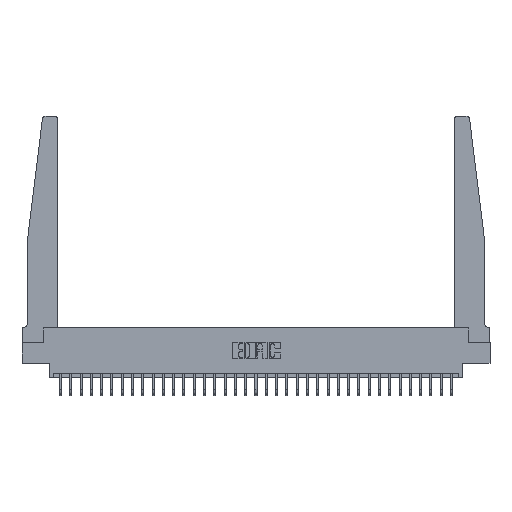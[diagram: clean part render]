
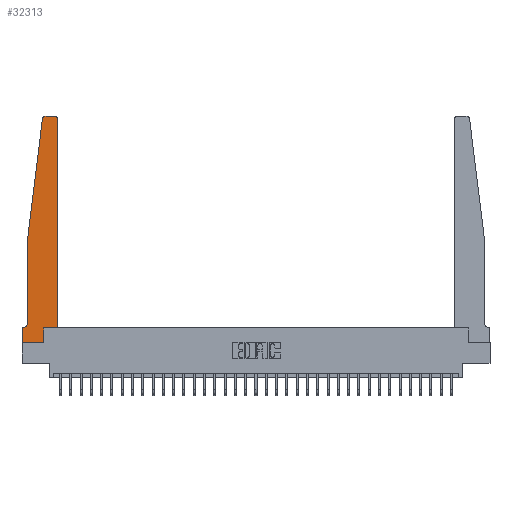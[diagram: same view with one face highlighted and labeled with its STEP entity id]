
A CAD part, top view. The second image highlights one B-rep face of the part: STEP entity #32313.
In plain terms, the highlighted planar face has unit normal (0, 0, 1).
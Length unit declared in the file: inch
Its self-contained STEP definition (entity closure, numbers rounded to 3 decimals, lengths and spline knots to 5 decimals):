
#9 = VECTOR ( 'NONE', #10334, 39.37008 ) ;
#131 = LINE ( 'NONE', #29189, #26053 ) ;
#541 = EDGE_CURVE ( 'NONE', #28573, #7818, #17181, .T. ) ;
#850 = VERTEX_POINT ( 'NONE', #10497 ) ;
#1174 = AXIS2_PLACEMENT_3D ( 'NONE', #7079, #29576, #24368 ) ;
#1526 = VERTEX_POINT ( 'NONE', #19208 ) ;
#2039 = CARTESIAN_POINT ( 'NONE',  ( 0.2605, 0.18, 0.37 ) ) ;
#2129 = LINE ( 'NONE', #14947, #18658 ) ;
#3239 = DIRECTION ( 'NONE',  ( 0., 0., -1. ) ) ;
#3535 = VECTOR ( 'NONE', #23952, 39.37008 ) ;
#4107 = VECTOR ( 'NONE', #19419, 39.37008 ) ;
#4383 = PLANE ( 'NONE',  #12985 ) ;
#4549 = DIRECTION ( 'NONE',  ( -0.122, -0.992, 0. ) ) ;
#4665 = CARTESIAN_POINT ( 'NONE',  ( 0.24675, 2.72367, 0.37 ) ) ;
#4707 = DIRECTION ( 'NONE',  ( 1., 0., 0. ) ) ;
#4791 = ORIENTED_EDGE ( 'NONE', *, *, #9170, .T. ) ;
#5146 = ORIENTED_EDGE ( 'NONE', *, *, #25690, .T. ) ;
#5312 = CIRCLE ( 'NONE', #24335, 0.05 ) ;
#5725 = VECTOR ( 'NONE', #4549, 39.37008 ) ;
#5954 = ORIENTED_EDGE ( 'NONE', *, *, #31740, .T. ) ;
#6059 = VERTEX_POINT ( 'NONE', #12554 ) ;
#6511 = EDGE_CURVE ( 'NONE', #10917, #8183, #19092, .T. ) ;
#7079 = CARTESIAN_POINT ( 'NONE',  ( 0.27653, 2.72, 0.37 ) ) ;
#7818 = VERTEX_POINT ( 'NONE', #21180 ) ;
#8036 = VERTEX_POINT ( 'NONE', #30176 ) ;
#8183 = VERTEX_POINT ( 'NONE', #31671 ) ;
#9170 = EDGE_CURVE ( 'NONE', #8183, #12860, #17336, .T. ) ;
#9410 = LINE ( 'NONE', #11577, #14124 ) ;
#9505 = ORIENTED_EDGE ( 'NONE', *, *, #6511, .T. ) ;
#9618 = CARTESIAN_POINT ( 'NONE',  ( 0.065, 1.25, 0.37 ) ) ;
#10334 = DIRECTION ( 'NONE',  ( 0., -1., 0. ) ) ;
#10497 = CARTESIAN_POINT ( 'NONE',  ( 0.015, 0.1875, 0.37 ) ) ;
#10652 = ORIENTED_EDGE ( 'NONE', *, *, #14332, .T. ) ;
#10917 = VERTEX_POINT ( 'NONE', #4665 ) ;
#11577 = CARTESIAN_POINT ( 'NONE',  ( 0., 0., 0.37 ) ) ;
#11601 = ORIENTED_EDGE ( 'NONE', *, *, #28352, .T. ) ;
#11802 = DIRECTION ( 'NONE',  ( 1., 0., 0. ) ) ;
#11889 = CARTESIAN_POINT ( 'NONE',  ( 0., 0., 0.37 ) ) ;
#12194 = DIRECTION ( 'NONE',  ( 1., 0., 0. ) ) ;
#12201 = ORIENTED_EDGE ( 'NONE', *, *, #29033, .T. ) ;
#12554 = CARTESIAN_POINT ( 'NONE',  ( 0., 0.1875, 0.37 ) ) ;
#12704 = LINE ( 'NONE', #2039, #4107 ) ;
#12860 = VERTEX_POINT ( 'NONE', #29856 ) ;
#12985 = AXIS2_PLACEMENT_3D ( 'NONE', #19627, #22109, #4707 ) ;
#13314 = CARTESIAN_POINT ( 'NONE',  ( 0.065, 0.1875, 0.37 ) ) ;
#13332 = DIRECTION ( 'NONE',  ( -1., 0., 0. ) ) ;
#13832 = ORIENTED_EDGE ( 'NONE', *, *, #28212, .T. ) ;
#14124 = VECTOR ( 'NONE', #11802, 39.37008 ) ;
#14144 = DIRECTION ( 'NONE',  ( -1., 0., 0. ) ) ;
#14332 = EDGE_CURVE ( 'NONE', #17943, #18675, #2129, .T. ) ;
#14537 = LINE ( 'NONE', #27121, #23931 ) ;
#14947 = CARTESIAN_POINT ( 'NONE',  ( 0.425, 0.18, 0.37 ) ) ;
#15581 = ORIENTED_EDGE ( 'NONE', *, *, #32252, .T. ) ;
#16327 = DIRECTION ( 'NONE',  ( 0., 0., 1. ) ) ;
#17181 = CIRCLE ( 'NONE', #32480, 0.03 ) ;
#17336 = LINE ( 'NONE', #9618, #26338 ) ;
#17438 = CARTESIAN_POINT ( 'NONE',  ( 0.425, 0.18, 0.37 ) ) ;
#17943 = VERTEX_POINT ( 'NONE', #28721 ) ;
#18658 = VECTOR ( 'NONE', #12194, 39.37008 ) ;
#18675 = VERTEX_POINT ( 'NONE', #17438 ) ;
#19092 = LINE ( 'NONE', #32127, #5725 ) ;
#19208 = CARTESIAN_POINT ( 'NONE',  ( 0.2605, 0., 0.37 ) ) ;
#19419 = DIRECTION ( 'NONE',  ( 0., 1., 0. ) ) ;
#19627 = CARTESIAN_POINT ( 'NONE',  ( 0., 0.1875, 0.37 ) ) ;
#20294 = ORIENTED_EDGE ( 'NONE', *, *, #541, .T. ) ;
#21180 = CARTESIAN_POINT ( 'NONE',  ( 0.395, 2.75, 0.37 ) ) ;
#21241 = LINE ( 'NONE', #25112, #9 ) ;
#22109 = DIRECTION ( 'NONE',  ( 0., 0., 1. ) ) ;
#22165 = CARTESIAN_POINT ( 'NONE',  ( 0.425, 2.72, 0.37 ) ) ;
#22396 = DIRECTION ( 'NONE',  ( 0., 1., 0. ) ) ;
#22517 = VERTEX_POINT ( 'NONE', #11889 ) ;
#22561 = ORIENTED_EDGE ( 'NONE', *, *, #28899, .T. ) ;
#23931 = VECTOR ( 'NONE', #22396, 39.37008 ) ;
#23952 = DIRECTION ( 'NONE',  ( -1., 0., 0. ) ) ;
#24335 = AXIS2_PLACEMENT_3D ( 'NONE', #28374, #3239, #13332 ) ;
#24368 = DIRECTION ( 'NONE',  ( 1., 0., 0. ) ) ;
#24822 = DIRECTION ( 'NONE',  ( 0., -1., 0. ) ) ;
#25112 = CARTESIAN_POINT ( 'NONE',  ( 0., 0., 0.37 ) ) ;
#25311 = EDGE_LOOP ( 'NONE', ( #15581, #22561, #9505, #4791, #5954, #13832, #5146, #11601, #30448, #10652, #12201, #20294 ) ) ;
#25690 = EDGE_CURVE ( 'NONE', #6059, #22517, #21241, .T. ) ;
#26053 = VECTOR ( 'NONE', #14144, 39.37008 ) ;
#26291 = CIRCLE ( 'NONE', #1174, 0.03 ) ;
#26338 = VECTOR ( 'NONE', #24822, 39.37008 ) ;
#26823 = CARTESIAN_POINT ( 'NONE',  ( 0.395, 2.72, 0.37 ) ) ;
#26923 = DIRECTION ( 'NONE',  ( 1., 0., 0. ) ) ;
#27121 = CARTESIAN_POINT ( 'NONE',  ( 0.425, 0.18, 0.37 ) ) ;
#28212 = EDGE_CURVE ( 'NONE', #850, #6059, #31461, .T. ) ;
#28352 = EDGE_CURVE ( 'NONE', #22517, #1526, #9410, .T. ) ;
#28374 = CARTESIAN_POINT ( 'NONE',  ( 0.015, 0.2375, 0.37 ) ) ;
#28573 = VERTEX_POINT ( 'NONE', #22165 ) ;
#28721 = CARTESIAN_POINT ( 'NONE',  ( 0.2605, 0.18, 0.37 ) ) ;
#28899 = EDGE_CURVE ( 'NONE', #8036, #10917, #26291, .T. ) ;
#29033 = EDGE_CURVE ( 'NONE', #18675, #28573, #14537, .T. ) ;
#29189 = CARTESIAN_POINT ( 'NONE',  ( 0.25, 2.75, 0.37 ) ) ;
#29576 = DIRECTION ( 'NONE',  ( 0., 0., 1. ) ) ;
#29856 = CARTESIAN_POINT ( 'NONE',  ( 0.065, 0.2375, 0.37 ) ) ;
#30176 = CARTESIAN_POINT ( 'NONE',  ( 0.27653, 2.75, 0.37 ) ) ;
#30427 = FACE_OUTER_BOUND ( 'NONE', #25311, .T. ) ;
#30448 = ORIENTED_EDGE ( 'NONE', *, *, #32309, .T. ) ;
#31461 = LINE ( 'NONE', #13314, #3535 ) ;
#31671 = CARTESIAN_POINT ( 'NONE',  ( 0.065, 1.25, 0.37 ) ) ;
#31740 = EDGE_CURVE ( 'NONE', #12860, #850, #5312, .T. ) ;
#32127 = CARTESIAN_POINT ( 'NONE',  ( 0.065, 1.25, 0.37 ) ) ;
#32252 = EDGE_CURVE ( 'NONE', #7818, #8036, #131, .T. ) ;
#32309 = EDGE_CURVE ( 'NONE', #1526, #17943, #12704, .T. ) ;
#32313 = ADVANCED_FACE ( 'NONE', ( #30427 ), #4383, .T. ) ;
#32480 = AXIS2_PLACEMENT_3D ( 'NONE', #26823, #16327, #26923 ) ;
